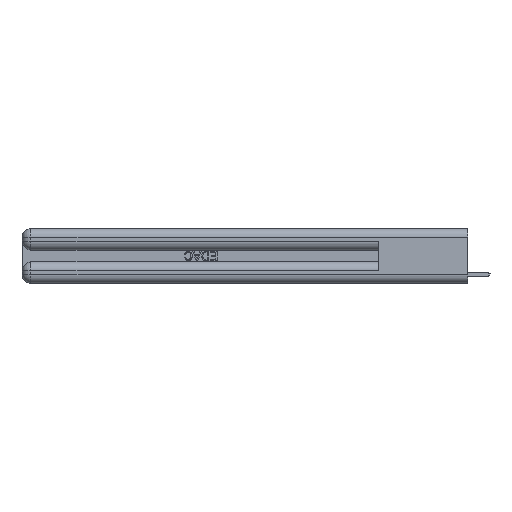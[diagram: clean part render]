
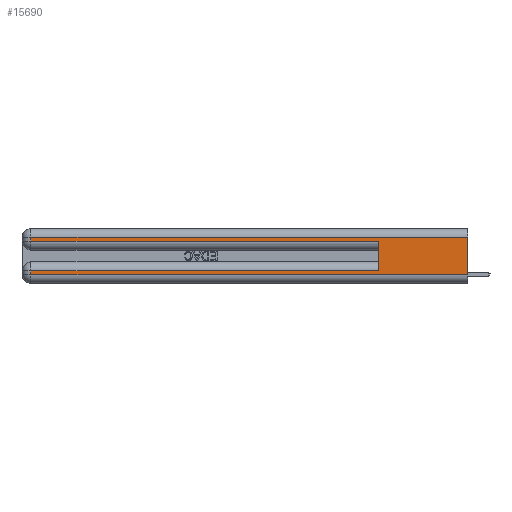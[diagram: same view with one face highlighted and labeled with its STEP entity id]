
A CAD part, left-side view. The second image highlights one B-rep face of the part: STEP entity #15690.
In plain terms, the highlighted planar face has unit normal (-1, 0, 0).
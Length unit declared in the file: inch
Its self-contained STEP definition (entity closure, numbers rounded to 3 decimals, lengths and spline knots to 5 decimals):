
#419 = LINE ( 'NONE', #26849, #2805 ) ;
#1096 = ORIENTED_EDGE ( 'NONE', *, *, #2571, .T. ) ;
#1301 = DIRECTION ( 'NONE',  ( 0., 0., -1. ) ) ;
#2571 = EDGE_CURVE ( 'NONE', #21236, #27088, #13617, .T. ) ;
#2577 = DIRECTION ( 'NONE',  ( 0., 1., 0. ) ) ;
#2805 = VECTOR ( 'NONE', #19416, 39.37008 ) ;
#2843 = CARTESIAN_POINT ( 'NONE',  ( 0., 0., 0.285 ) ) ;
#3021 = EDGE_CURVE ( 'NONE', #4753, #13658, #20274, .T. ) ;
#4137 = VECTOR ( 'NONE', #10276, 39.37008 ) ;
#4297 = CARTESIAN_POINT ( 'NONE',  ( 0., 2.94, 0.31 ) ) ;
#4753 = VERTEX_POINT ( 'NONE', #20764 ) ;
#4969 = EDGE_CURVE ( 'NONE', #4753, #27088, #5384, .T. ) ;
#5384 = LINE ( 'NONE', #16381, #23113 ) ;
#5707 = VECTOR ( 'NONE', #24840, 39.37008 ) ;
#6778 = EDGE_CURVE ( 'NONE', #7512, #6959, #25351, .T. ) ;
#6959 = VERTEX_POINT ( 'NONE', #23497 ) ;
#7512 = VERTEX_POINT ( 'NONE', #15163 ) ;
#8278 = CARTESIAN_POINT ( 'NONE',  ( 0., 0.6, 0.145 ) ) ;
#8489 = AXIS2_PLACEMENT_3D ( 'NONE', #8580, #18767, #1301 ) ;
#8490 = EDGE_CURVE ( 'NONE', #6959, #21236, #419, .T. ) ;
#8580 = CARTESIAN_POINT ( 'NONE',  ( 0., 0., 0.37 ) ) ;
#10276 = DIRECTION ( 'NONE',  ( 0., -1., 0. ) ) ;
#10566 = ORIENTED_EDGE ( 'NONE', *, *, #25567, .T. ) ;
#11104 = CARTESIAN_POINT ( 'NONE',  ( 0., 0., 0.06 ) ) ;
#11162 = DIRECTION ( 'NONE',  ( 0., 0., -1. ) ) ;
#11246 = LINE ( 'NONE', #2843, #4137 ) ;
#12515 = CARTESIAN_POINT ( 'NONE',  ( 0., 2.94, 0.285 ) ) ;
#13617 = LINE ( 'NONE', #11104, #19515 ) ;
#13658 = VERTEX_POINT ( 'NONE', #4297 ) ;
#14221 = VERTEX_POINT ( 'NONE', #16749 ) ;
#14948 = ORIENTED_EDGE ( 'NONE', *, *, #15003, .F. ) ;
#15003 = EDGE_CURVE ( 'NONE', #7512, #14221, #19648, .T. ) ;
#15163 = CARTESIAN_POINT ( 'NONE',  ( 0., 0.6, 0.085 ) ) ;
#15185 = VECTOR ( 'NONE', #17289, 39.37008 ) ;
#15196 = CARTESIAN_POINT ( 'NONE',  ( 0., 0., 0.31 ) ) ;
#15690 = ADVANCED_FACE ( 'NONE', ( #19173 ), #26095, .F. ) ;
#16130 = EDGE_CURVE ( 'NONE', #13658, #22745, #17969, .T. ) ;
#16381 = CARTESIAN_POINT ( 'NONE',  ( 0., 0., 0.37 ) ) ;
#16749 = CARTESIAN_POINT ( 'NONE',  ( 0., 0.6, 0.285 ) ) ;
#17289 = DIRECTION ( 'NONE',  ( 0., 1., 0. ) ) ;
#17441 = CARTESIAN_POINT ( 'NONE',  ( 0., 2.94, 0.06 ) ) ;
#17744 = CARTESIAN_POINT ( 'NONE',  ( 0., 2.94, 0.37 ) ) ;
#17969 = LINE ( 'NONE', #17744, #5707 ) ;
#18767 = DIRECTION ( 'NONE',  ( 1., 0., 0. ) ) ;
#19173 = FACE_OUTER_BOUND ( 'NONE', #31807, .T. ) ;
#19416 = DIRECTION ( 'NONE',  ( 0., 0., -1. ) ) ;
#19515 = VECTOR ( 'NONE', #25807, 39.37008 ) ;
#19648 = LINE ( 'NONE', #8278, #22365 ) ;
#20031 = ORIENTED_EDGE ( 'NONE', *, *, #6778, .T. ) ;
#20274 = LINE ( 'NONE', #15196, #25321 ) ;
#20764 = CARTESIAN_POINT ( 'NONE',  ( 0., 0., 0.31 ) ) ;
#20986 = ORIENTED_EDGE ( 'NONE', *, *, #8490, .T. ) ;
#21236 = VERTEX_POINT ( 'NONE', #17441 ) ;
#22365 = VECTOR ( 'NONE', #25903, 39.37008 ) ;
#22745 = VERTEX_POINT ( 'NONE', #12515 ) ;
#23113 = VECTOR ( 'NONE', #11162, 39.37008 ) ;
#23497 = CARTESIAN_POINT ( 'NONE',  ( 0., 2.94, 0.085 ) ) ;
#23707 = ORIENTED_EDGE ( 'NONE', *, *, #4969, .F. ) ;
#24840 = DIRECTION ( 'NONE',  ( 0., 0., -1. ) ) ;
#25321 = VECTOR ( 'NONE', #2577, 39.37008 ) ;
#25351 = LINE ( 'NONE', #27587, #15185 ) ;
#25567 = EDGE_CURVE ( 'NONE', #22745, #14221, #11246, .T. ) ;
#25807 = DIRECTION ( 'NONE',  ( 0., -1., 0. ) ) ;
#25903 = DIRECTION ( 'NONE',  ( 0., 0., 1. ) ) ;
#26095 = PLANE ( 'NONE',  #8489 ) ;
#26555 = CARTESIAN_POINT ( 'NONE',  ( 0., 0., 0.06 ) ) ;
#26849 = CARTESIAN_POINT ( 'NONE',  ( 0., 2.94, 0.37 ) ) ;
#27088 = VERTEX_POINT ( 'NONE', #26555 ) ;
#27587 = CARTESIAN_POINT ( 'NONE',  ( 0., 0., 0.085 ) ) ;
#29333 = ORIENTED_EDGE ( 'NONE', *, *, #3021, .T. ) ;
#31807 = EDGE_LOOP ( 'NONE', ( #23707, #29333, #32448, #10566, #14948, #20031, #20986, #1096 ) ) ;
#32448 = ORIENTED_EDGE ( 'NONE', *, *, #16130, .T. ) ;
